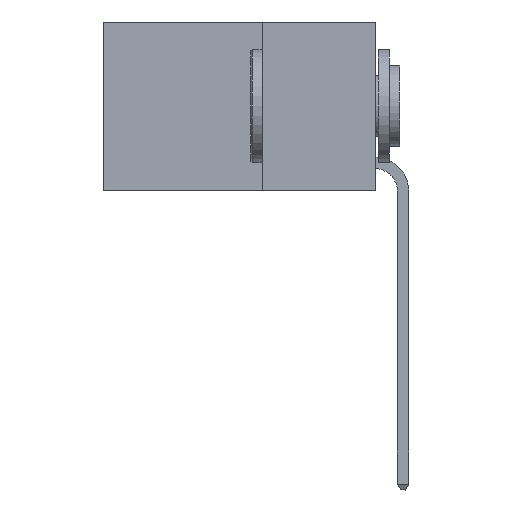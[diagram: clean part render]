
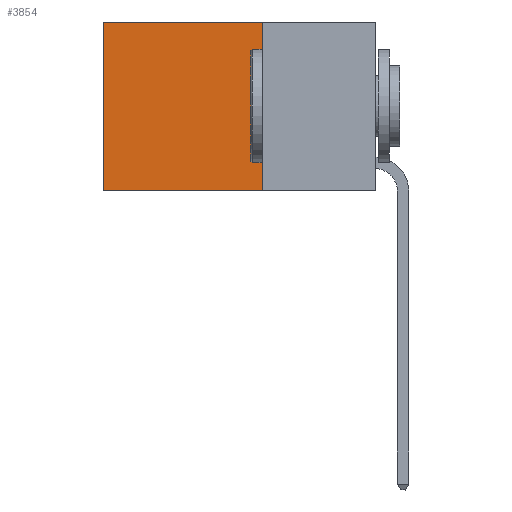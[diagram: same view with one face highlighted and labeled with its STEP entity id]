
A CAD part, left-side view. The second image highlights one B-rep face of the part: STEP entity #3854.
In plain terms, the highlighted planar face has unit normal (-1, 0, 0).
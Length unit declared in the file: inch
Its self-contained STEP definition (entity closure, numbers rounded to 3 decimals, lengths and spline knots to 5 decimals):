
#364 = FACE_OUTER_BOUND ( 'NONE', #18171, .T. ) ;
#729 = CARTESIAN_POINT ( 'NONE',  ( 0.2625, 0.25, -0.37 ) ) ;
#3854 = ADVANCED_FACE ( 'NONE', ( #364 ), #4637, .F. ) ;
#3925 = VERTEX_POINT ( 'NONE', #12946 ) ;
#4038 = ORIENTED_EDGE ( 'NONE', *, *, #21876, .F. ) ;
#4121 = CARTESIAN_POINT ( 'NONE',  ( 0.2625, 0.25, -0.37 ) ) ;
#4637 = PLANE ( 'NONE',  #7037 ) ;
#5269 = VERTEX_POINT ( 'NONE', #10758 ) ;
#5315 = EDGE_CURVE ( 'NONE', #5269, #3925, #19565, .T. ) ;
#5633 = ORIENTED_EDGE ( 'NONE', *, *, #5315, .T. ) ;
#7037 = AXIS2_PLACEMENT_3D ( 'NONE', #10057, #17760, #13764 ) ;
#7149 = DIRECTION ( 'NONE',  ( 0., 0., -1. ) ) ;
#7811 = ORIENTED_EDGE ( 'NONE', *, *, #23614, .F. ) ;
#8986 = VECTOR ( 'NONE', #11802, 39.37008 ) ;
#9530 = CARTESIAN_POINT ( 'NONE',  ( 0.2625, 0.25, 0. ) ) ;
#10057 = CARTESIAN_POINT ( 'NONE',  ( 0.2625, 0.25, 0. ) ) ;
#10329 = LINE ( 'NONE', #17548, #13870 ) ;
#10576 = VERTEX_POINT ( 'NONE', #729 ) ;
#10706 = ORIENTED_EDGE ( 'NONE', *, *, #24242, .T. ) ;
#10758 = CARTESIAN_POINT ( 'NONE',  ( 0.2625, 0.6, 0. ) ) ;
#11802 = DIRECTION ( 'NONE',  ( 0., 1., 0. ) ) ;
#12243 = DIRECTION ( 'NONE',  ( 0., 0., -1. ) ) ;
#12946 = CARTESIAN_POINT ( 'NONE',  ( 0.2625, 0.6, -0.37 ) ) ;
#13718 = LINE ( 'NONE', #4121, #8986 ) ;
#13764 = DIRECTION ( 'NONE',  ( 0., 0., -1. ) ) ;
#13870 = VECTOR ( 'NONE', #18033, 39.37008 ) ;
#17548 = CARTESIAN_POINT ( 'NONE',  ( 0.2625, 0.25, 0. ) ) ;
#17760 = DIRECTION ( 'NONE',  ( 1., 0., 0. ) ) ;
#17923 = CARTESIAN_POINT ( 'NONE',  ( 0.2625, 0.6, 0. ) ) ;
#18033 = DIRECTION ( 'NONE',  ( 0., 1., 0. ) ) ;
#18171 = EDGE_LOOP ( 'NONE', ( #5633, #4038, #7811, #10706 ) ) ;
#19565 = LINE ( 'NONE', #17923, #22362 ) ;
#20730 = LINE ( 'NONE', #23070, #21029 ) ;
#21029 = VECTOR ( 'NONE', #7149, 39.37008 ) ;
#21792 = VERTEX_POINT ( 'NONE', #9530 ) ;
#21876 = EDGE_CURVE ( 'NONE', #10576, #3925, #13718, .T. ) ;
#22362 = VECTOR ( 'NONE', #12243, 39.37008 ) ;
#23070 = CARTESIAN_POINT ( 'NONE',  ( 0.2625, 0.25, 0. ) ) ;
#23614 = EDGE_CURVE ( 'NONE', #21792, #10576, #20730, .T. ) ;
#24242 = EDGE_CURVE ( 'NONE', #21792, #5269, #10329, .T. ) ;
